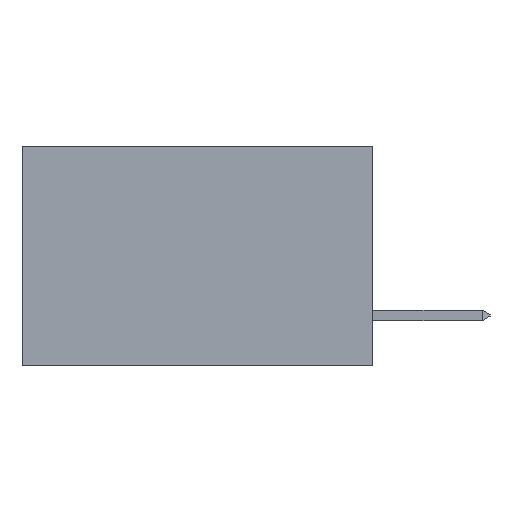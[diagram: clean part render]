
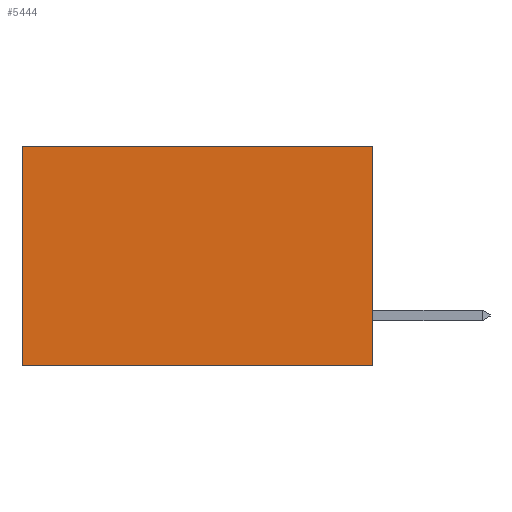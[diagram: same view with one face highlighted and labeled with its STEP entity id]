
A CAD part, left-side view. The second image highlights one B-rep face of the part: STEP entity #5444.
In plain terms, the highlighted planar face has unit normal (-1, 0, 0).
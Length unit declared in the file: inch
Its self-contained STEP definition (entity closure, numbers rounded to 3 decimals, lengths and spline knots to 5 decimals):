
#1791 = DIRECTION ( 'NONE',  ( 0., 1., 0. ) ) ;
#1969 = CARTESIAN_POINT ( 'NONE',  ( 0.277, 0., 0. ) ) ;
#3925 = DIRECTION ( 'NONE',  ( 0., 1., 0. ) ) ;
#4095 = VECTOR ( 'NONE', #18436, 39.37008 ) ;
#4178 = ORIENTED_EDGE ( 'NONE', *, *, #25683, .T. ) ;
#4715 = CARTESIAN_POINT ( 'NONE',  ( 0.277, 0.59, -0.37 ) ) ;
#5444 = ADVANCED_FACE ( 'NONE', ( #7369 ), #11749, .F. ) ;
#5559 = VERTEX_POINT ( 'NONE', #4715 ) ;
#5750 = DIRECTION ( 'NONE',  ( 0., 0., -1. ) ) ;
#6049 = EDGE_CURVE ( 'NONE', #27264, #26599, #25127, .T. ) ;
#6848 = ORIENTED_EDGE ( 'NONE', *, *, #14084, .F. ) ;
#7369 = FACE_OUTER_BOUND ( 'NONE', #23778, .T. ) ;
#9278 = CARTESIAN_POINT ( 'NONE',  ( 0.277, 0.59, 0. ) ) ;
#10706 = LINE ( 'NONE', #16209, #4095 ) ;
#11749 = PLANE ( 'NONE',  #23828 ) ;
#12053 = VECTOR ( 'NONE', #5750, 39.37008 ) ;
#12111 = DIRECTION ( 'NONE',  ( 0., 0., -1. ) ) ;
#12264 = DIRECTION ( 'NONE',  ( 1., 0., 0. ) ) ;
#12325 = CARTESIAN_POINT ( 'NONE',  ( 0.277, 0., -0.37 ) ) ;
#13804 = ORIENTED_EDGE ( 'NONE', *, *, #19434, .F. ) ;
#14084 = EDGE_CURVE ( 'NONE', #15940, #5559, #15558, .T. ) ;
#14656 = VECTOR ( 'NONE', #1791, 39.37008 ) ;
#15043 = CARTESIAN_POINT ( 'NONE',  ( 0.277, 0., -0.37 ) ) ;
#15558 = LINE ( 'NONE', #15043, #20782 ) ;
#15940 = VERTEX_POINT ( 'NONE', #21094 ) ;
#16209 = CARTESIAN_POINT ( 'NONE',  ( 0.277, 0., -0.37 ) ) ;
#16904 = CARTESIAN_POINT ( 'NONE',  ( 0.277, 0.59, -0.37 ) ) ;
#18436 = DIRECTION ( 'NONE',  ( 0., 0., -1. ) ) ;
#18682 = LINE ( 'NONE', #16904, #12053 ) ;
#19434 = EDGE_CURVE ( 'NONE', #27264, #15940, #10706, .T. ) ;
#20782 = VECTOR ( 'NONE', #3925, 39.37008 ) ;
#21094 = CARTESIAN_POINT ( 'NONE',  ( 0.277, 0., -0.37 ) ) ;
#23778 = EDGE_LOOP ( 'NONE', ( #4178, #6848, #13804, #26037 ) ) ;
#23828 = AXIS2_PLACEMENT_3D ( 'NONE', #12325, #12264, #12111 ) ;
#24979 = CARTESIAN_POINT ( 'NONE',  ( 0.277, 0., 0. ) ) ;
#25127 = LINE ( 'NONE', #1969, #14656 ) ;
#25683 = EDGE_CURVE ( 'NONE', #26599, #5559, #18682, .T. ) ;
#26037 = ORIENTED_EDGE ( 'NONE', *, *, #6049, .T. ) ;
#26599 = VERTEX_POINT ( 'NONE', #9278 ) ;
#27264 = VERTEX_POINT ( 'NONE', #24979 ) ;
